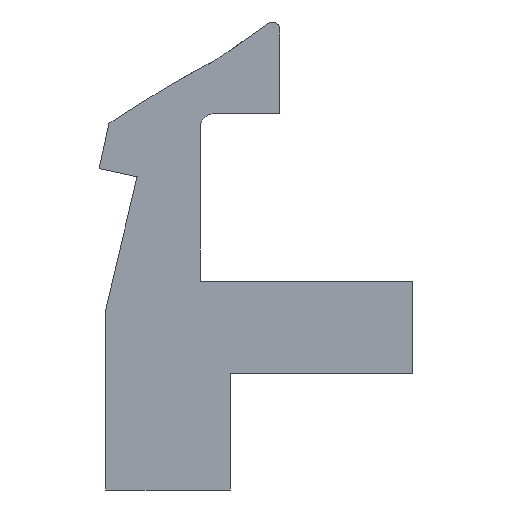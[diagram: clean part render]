
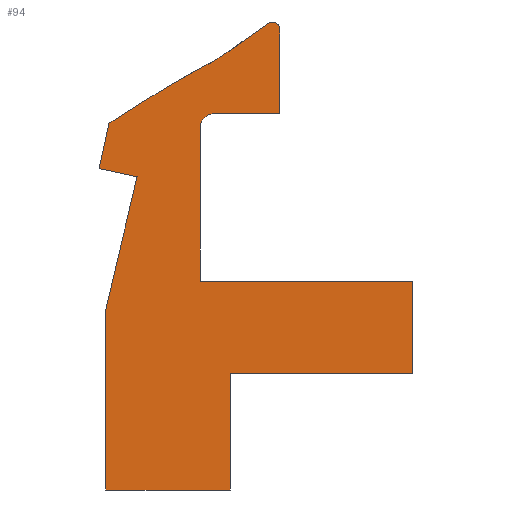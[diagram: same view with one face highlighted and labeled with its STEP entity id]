
A CAD part, front view. The second image highlights one B-rep face of the part: STEP entity #94.
In plain terms, the highlighted planar face has unit normal (0, -1, 0).
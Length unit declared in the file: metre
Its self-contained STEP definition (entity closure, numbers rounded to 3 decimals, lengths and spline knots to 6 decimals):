
#94=ADVANCED_FACE('18:24',(#188),#189,.F.);
#188=FACE_OUTER_BOUND('',#1390,.T.);
#189=PLANE('',#1391);
#1390=EDGE_LOOP('',(#1725,#1726,#1727,#1728,#1729,#1730,#1731,#1732,#1733,#1734,#1735,#1736,#1737,#1738,#1739,#1740,#1741,#1742,#1743,#1744,#1745));
#1391=AXIS2_PLACEMENT_3D('',#1746,#1747,#1748);
#1725=ORIENTED_EDGE('',*,*,#1880,.T.);
#1726=ORIENTED_EDGE('',*,*,#1878,.F.);
#1727=ORIENTED_EDGE('',*,*,#1885,.F.);
#1728=ORIENTED_EDGE('',*,*,#1851,.F.);
#1729=ORIENTED_EDGE('',*,*,#1775,.F.);
#1730=ORIENTED_EDGE('',*,*,#1850,.F.);
#1731=ORIENTED_EDGE('',*,*,#1846,.T.);
#1732=ORIENTED_EDGE('',*,*,#1843,.F.);
#1733=ORIENTED_EDGE('',*,*,#1779,.F.);
#1734=ORIENTED_EDGE('',*,*,#1841,.T.);
#1735=ORIENTED_EDGE('',*,*,#1797,.F.);
#1736=ORIENTED_EDGE('',*,*,#1817,.F.);
#1737=ORIENTED_EDGE('',*,*,#1818,.F.);
#1738=ORIENTED_EDGE('',*,*,#1795,.F.);
#1739=ORIENTED_EDGE('',*,*,#1856,.F.);
#1740=ORIENTED_EDGE('',*,*,#1858,.F.);
#1741=ORIENTED_EDGE('',*,*,#1886,.F.);
#1742=ORIENTED_EDGE('',*,*,#1871,.F.);
#1743=ORIENTED_EDGE('',*,*,#1861,.T.);
#1744=ORIENTED_EDGE('',*,*,#1872,.F.);
#1745=ORIENTED_EDGE('',*,*,#1865,.T.);
#1746=CARTESIAN_POINT('',(0.000691,-0.01,0.018046));
#1747=DIRECTION('',(0.,1.0,0.));
#1748=DIRECTION('',(0.214,0.,0.977));
#1775=EDGE_CURVE('20:6809',#1908,#1904,#1910,.F.);
#1779=EDGE_CURVE('18:89',#1916,#1912,#1918,.F.);
#1795=EDGE_CURVE('18:113',#1948,#1944,#1950,.F.);
#1797=EDGE_CURVE('19:5096',#1951,#1954,#1955,.F.);
#1817=EDGE_CURVE('19:5096',#1984,#1951,#1986,.F.);
#1818=EDGE_CURVE('18:113',#1944,#1984,#1987,.F.);
#1841=EDGE_CURVE('18:101',#1916,#1954,#2020,.F.);
#1843=EDGE_CURVE('18:89',#1912,#2022,#2023,.F.);
#1846=EDGE_CURVE('18:146',#2027,#2022,#2028,.F.);
#1850=EDGE_CURVE('18:143',#2027,#1908,#2033,.F.);
#1851=EDGE_CURVE('20:6809',#1904,#2034,#2035,.F.);
#1856=EDGE_CURVE('18:119',#2041,#1948,#2043,.T.);
#1858=EDGE_CURVE('18:122',#2044,#2041,#2047,.F.);
#1861=EDGE_CURVE('20:771',#2052,#2049,#2053,.F.);
#1865=EDGE_CURVE('20:774',#2060,#2058,#2061,.F.);
#1871=EDGE_CURVE('18:128',#2052,#2067,#2070,.T.);
#1872=EDGE_CURVE('20:809',#2060,#2049,#2071,.F.);
#1878=EDGE_CURVE('18:137',#2079,#2074,#2081,.F.);
#1880=EDGE_CURVE('18:134',#2058,#2074,#2083,.T.);
#1885=EDGE_CURVE('18:140',#2034,#2079,#2088,.F.);
#1886=EDGE_CURVE('18:125',#2067,#2044,#2089,.T.);
#1904=VERTEX_POINT('',#2111);
#1908=VERTEX_POINT('',#2116);
#1910=CIRCLE('',#2119,0.0006);
#1912=VERTEX_POINT('',#2121);
#1916=VERTEX_POINT('',#2126);
#1918=CIRCLE('',#2129,0.0003);
#1944=VERTEX_POINT('',#2191);
#1948=VERTEX_POINT('',#2196);
#1950=CIRCLE('',#2199,0.0535);
#1951=VERTEX_POINT('',#2200);
#1954=VERTEX_POINT('',#2204);
#1955=CIRCLE('',#2205,0.00366);
#1984=VERTEX_POINT('',#2279);
#1986=CIRCLE('',#2282,0.00366);
#1987=CIRCLE('',#2283,0.0535);
#2020=LINE('',#2356,#2357);
#2022=VERTEX_POINT('',#2360);
#2023=CIRCLE('',#2361,0.0003);
#2027=VERTEX_POINT('',#2366);
#2028=LINE('',#2367,#2368);
#2033=LINE('',#2376,#2377);
#2034=VERTEX_POINT('',#2378);
#2035=CIRCLE('',#2379,0.0006);
#2041=VERTEX_POINT('',#2387);
#2043=LINE('',#2390,#2391);
#2044=VERTEX_POINT('',#2392);
#2047=LINE('',#2396,#2397);
#2049=VERTEX_POINT('',#2400);
#2052=VERTEX_POINT('',#2404);
#2053=LINE('',#2405,#2406);
#2058=VERTEX_POINT('',#2413);
#2060=VERTEX_POINT('',#2416);
#2061=LINE('',#2417,#2418);
#2067=VERTEX_POINT('',#2426);
#2070=LINE('',#2431,#2432);
#2071=LINE('',#2433,#2434);
#2074=VERTEX_POINT('',#2438);
#2079=VERTEX_POINT('',#2445);
#2081=LINE('',#2448,#2449);
#2083=LINE('',#2451,#2452);
#2088=LINE('',#2460,#2461);
#2089=LINE('',#2462,#2463);
#2111=CARTESIAN_POINT('',(0.004245,-0.01,0.020034));
#2116=CARTESIAN_POINT('',(0.004669,-0.01,0.02021));
#2119=AXIS2_PLACEMENT_3D('',#2485,#2486,#2487);
#2121=CARTESIAN_POINT('',(0.007329,-0.01,0.024128));
#2126=CARTESIAN_POINT('',(0.007018,-0.01,0.024108));
#2129=AXIS2_PLACEMENT_3D('',#2493,#2494,#2495);
#2191=CARTESIAN_POINT('',(0.002793,-0.01,0.021444));
#2196=CARTESIAN_POINT('',(0.000135,-0.01,0.019787));
#2199=AXIS2_PLACEMENT_3D('',#2513,#2514,#2515);
#2200=CARTESIAN_POINT('',(0.004815,-0.01,0.022574));
#2204=CARTESIAN_POINT('',(0.005001,-0.01,0.022696));
#2205=AXIS2_PLACEMENT_3D('',#2517,#2518,#2519);
#2279=CARTESIAN_POINT('',(0.004622,-0.01,0.022464));
#2282=AXIS2_PLACEMENT_3D('',#2544,#2545,#2546);
#2283=AXIS2_PLACEMENT_3D('',#2547,#2548,#2549);
#2356=CARTESIAN_POINT('',(0.003872,-0.01,0.021906));
#2357=VECTOR('',#2575,1.0);
#2360=CARTESIAN_POINT('',(0.00749,-0.01,0.023862));
#2361=AXIS2_PLACEMENT_3D('',#2577,#2578,#2579);
#2366=CARTESIAN_POINT('',(0.00749,-0.01,0.02021));
#2367=CARTESIAN_POINT('',(0.00749,-0.01,0.018509));
#2368=VECTOR('',#2584,1.0);
#2376=CARTESIAN_POINT('',(0.000345,-0.01,0.02021));
#2377=VECTOR('',#2588,1.0);
#2378=CARTESIAN_POINT('',(0.004069,-0.01,0.01961));
#2379=AXIS2_PLACEMENT_3D('',#2589,#2590,#2591);
#2387=CARTESIAN_POINT('',(-0.00029,-0.01,0.017847));
#2390=CARTESIAN_POINT('',(-0.000139,-0.01,0.018533));
#2391=VECTOR('',#2598,1.0);
#2392=CARTESIAN_POINT('',(0.001348,-0.01,0.017488));
#2396=CARTESIAN_POINT('',(0.00054,-0.01,0.017665));
#2397=VECTOR('',#2600,1.0);
#2400=CARTESIAN_POINT('',(0.005368,-0.01,0.004));
#2404=CARTESIAN_POINT('',(0.0,-0.01,0.004));
#2405=CARTESIAN_POINT('',(0.000345,-0.01,0.004));
#2406=VECTOR('',#2603,1.0);
#2413=CARTESIAN_POINT('',(0.013231,-0.01,0.009));
#2416=CARTESIAN_POINT('',(0.005368,-0.01,0.009));
#2417=CARTESIAN_POINT('',(0.000345,-0.01,0.009));
#2418=VECTOR('',#2607,1.0);
#2426=CARTESIAN_POINT('',(0.,-0.01,0.011791));
#2431=CARTESIAN_POINT('',(0.0,-0.01,0.0));
#2432=VECTOR('',#2615,1.0);
#2433=CARTESIAN_POINT('',(0.005368,-0.01,0.013523));
#2434=VECTOR('',#2616,1.0);
#2438=CARTESIAN_POINT('',(0.013231,-0.01,0.013));
#2445=CARTESIAN_POINT('',(0.004069,-0.01,0.013));
#2448=CARTESIAN_POINT('',(0.002845,-0.01,0.013));
#2449=VECTOR('',#2624,1.0);
#2451=CARTESIAN_POINT('',(0.013231,-0.01,0.008523));
#2452=VECTOR('',#2628,1.0);
#2460=CARTESIAN_POINT('',(0.004069,-0.01,0.019273));
#2461=VECTOR('',#2635,0.01);
#2462=CARTESIAN_POINT('',(0.,-0.01,0.011791));
#2463=VECTOR('',#2636,1.);
#2485=CARTESIAN_POINT('',(0.004669,-0.01,0.01961));
#2486=DIRECTION('',(0.,1.0,0.));
#2487=DIRECTION('',(-0.707,0.,0.707));
#2493=CARTESIAN_POINT('',(0.00719,-0.01,0.023862));
#2494=DIRECTION('',(0.,-1.0,0.));
#2495=DIRECTION('',(0.462,0.,0.887));
#2513=CARTESIAN_POINT('',(0.029755,-0.01,-0.024765));
#2514=DIRECTION('',(0.,-1.0,0.));
#2515=DIRECTION('',(-0.504,0.,0.864));
#2517=CARTESIAN_POINT('',(0.002903,-0.01,0.025695));
#2518=DIRECTION('',(0.,1.0,0.));
#2519=DIRECTION('',(0.523,0.,-0.853));
#2544=CARTESIAN_POINT('',(0.002903,-0.01,0.025695));
#2545=DIRECTION('',(0.,1.0,0.));
#2546=DIRECTION('',(0.523,0.,-0.853));
#2547=CARTESIAN_POINT('',(0.029755,-0.01,-0.024765));
#2548=DIRECTION('',(0.,-1.0,0.));
#2549=DIRECTION('',(-0.504,0.,0.864));
#2575=DIRECTION('',(0.819,0.,0.573));
#2577=CARTESIAN_POINT('',(0.00719,-0.01,0.023862));
#2578=DIRECTION('',(0.,-1.0,0.));
#2579=DIRECTION('',(0.462,0.,0.887));
#2584=DIRECTION('',(0.,0.,-1.0));
#2588=DIRECTION('',(1.0,0.,0.));
#2589=CARTESIAN_POINT('',(0.004669,-0.01,0.01961));
#2590=DIRECTION('',(0.,1.0,0.));
#2591=DIRECTION('',(-0.707,0.,0.707));
#2598=DIRECTION('',(0.214,0.0,0.977));
#2600=DIRECTION('',(0.977,0.,-0.214));
#2603=DIRECTION('',(-1.0,0.,0.0));
#2607=DIRECTION('',(-1.0,0.,0.0));
#2615=DIRECTION('',(0.0,0.0,1.0));
#2616=DIRECTION('',(0.0,0.,1.0));
#2624=DIRECTION('',(-1.0,0.,0.0));
#2628=DIRECTION('',(0.,0.,1.0));
#2635=DIRECTION('',(0.0,0.,1.0));
#2636=DIRECTION('',(0.23,0.0,0.973));
